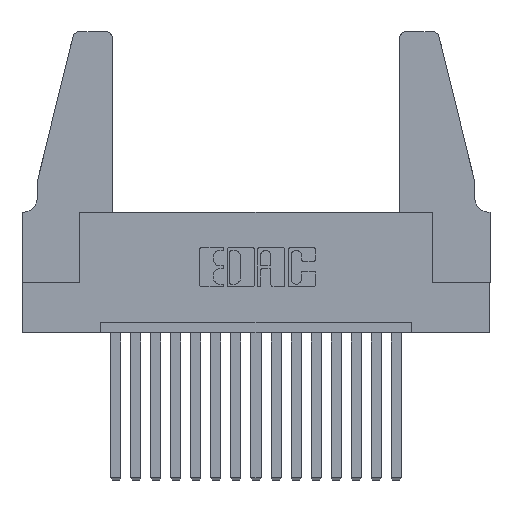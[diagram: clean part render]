
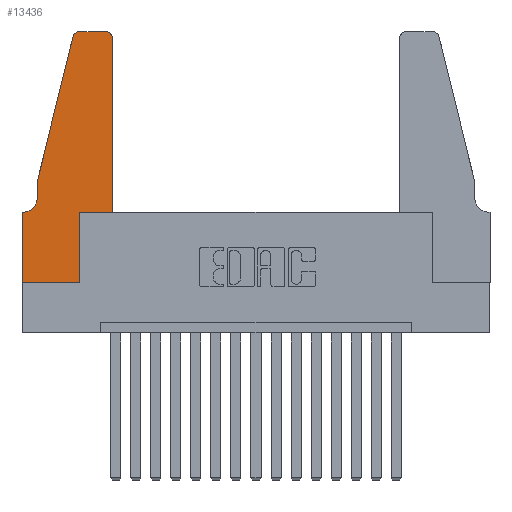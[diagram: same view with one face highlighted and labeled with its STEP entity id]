
A CAD part, top view. The second image highlights one B-rep face of the part: STEP entity #13436.
In plain terms, the highlighted planar face has unit normal (0, 0, 1).
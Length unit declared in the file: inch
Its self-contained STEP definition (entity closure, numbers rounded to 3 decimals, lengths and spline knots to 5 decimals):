
#142 = PLANE ( 'NONE',  #14912 ) ;
#301 = VERTEX_POINT ( 'NONE', #14000 ) ;
#553 = DIRECTION ( 'NONE',  ( 1., 0., 0. ) ) ;
#566 = ORIENTED_EDGE ( 'NONE', *, *, #6443, .T. ) ;
#1044 = DIRECTION ( 'NONE',  ( 1., 0., 0. ) ) ;
#1293 = VECTOR ( 'NONE', #553, 39.37008 ) ;
#1492 = VECTOR ( 'NONE', #10467, 39.37008 ) ;
#1547 = ORIENTED_EDGE ( 'NONE', *, *, #10667, .T. ) ;
#1606 = VECTOR ( 'NONE', #9524, 39.37008 ) ;
#1915 = LINE ( 'NONE', #5362, #1293 ) ;
#1996 = ORIENTED_EDGE ( 'NONE', *, *, #5969, .T. ) ;
#2199 = EDGE_CURVE ( 'NONE', #10345, #11494, #12308, .T. ) ;
#2483 = DIRECTION ( 'NONE',  ( 0., 0., -1. ) ) ;
#2499 = CARTESIAN_POINT ( 'NONE',  ( 0.2865, 0.35, 0.37 ) ) ;
#2780 = VERTEX_POINT ( 'NONE', #6485 ) ;
#2824 = CARTESIAN_POINT ( 'NONE',  ( 0.2865, 0.35, 0.37 ) ) ;
#2890 = CARTESIAN_POINT ( 'NONE',  ( 0.0755, 0.5, 0.37 ) ) ;
#3050 = EDGE_CURVE ( 'NONE', #11494, #301, #12895, .T. ) ;
#3321 = VECTOR ( 'NONE', #12921, 39.37008 ) ;
#3892 = VERTEX_POINT ( 'NONE', #12798 ) ;
#4064 = EDGE_CURVE ( 'NONE', #10422, #14339, #14464, .T. ) ;
#4308 = CARTESIAN_POINT ( 'NONE',  ( 0.2605, 1.25, 0.37 ) ) ;
#4333 = VECTOR ( 'NONE', #6754, 39.37008 ) ;
#4373 = CARTESIAN_POINT ( 'NONE',  ( 0., 0., 0.37 ) ) ;
#4433 = CARTESIAN_POINT ( 'NONE',  ( 0.0755, 0.35, 0.37 ) ) ;
#4600 = DIRECTION ( 'NONE',  ( 1., 0., 0. ) ) ;
#4766 = DIRECTION ( 'NONE',  ( 0., 0., 1. ) ) ;
#5066 = LINE ( 'NONE', #4308, #1606 ) ;
#5111 = EDGE_CURVE ( 'NONE', #3892, #8811, #5066, .T. ) ;
#5274 = EDGE_LOOP ( 'NONE', ( #10305, #7684, #6700, #5929, #566, #9186, #1996, #10435, #7729, #9344, #14558, #1547 ) ) ;
#5362 = CARTESIAN_POINT ( 'NONE',  ( 0., 0., 0.37 ) ) ;
#5525 = LINE ( 'NONE', #12229, #12070 ) ;
#5929 = ORIENTED_EDGE ( 'NONE', *, *, #3050, .T. ) ;
#5969 = EDGE_CURVE ( 'NONE', #14339, #2780, #11588, .T. ) ;
#6137 = CARTESIAN_POINT ( 'NONE',  ( 0.284, 1.25, 0.37 ) ) ;
#6207 = DIRECTION ( 'NONE',  ( 0., -1., 0. ) ) ;
#6263 = AXIS2_PLACEMENT_3D ( 'NONE', #7651, #6409, #1044 ) ;
#6409 = DIRECTION ( 'NONE',  ( 0., 0., 1. ) ) ;
#6429 = AXIS2_PLACEMENT_3D ( 'NONE', #16488, #4766, #4600 ) ;
#6443 = EDGE_CURVE ( 'NONE', #301, #10422, #11151, .T. ) ;
#6485 = CARTESIAN_POINT ( 'NONE',  ( 0., 0., 0.37 ) ) ;
#6700 = ORIENTED_EDGE ( 'NONE', *, *, #2199, .T. ) ;
#6754 = DIRECTION ( 'NONE',  ( 0., -1., 0. ) ) ;
#6848 = EDGE_CURVE ( 'NONE', #2780, #15087, #1915, .T. ) ;
#7066 = EDGE_CURVE ( 'NONE', #8811, #10345, #10366, .T. ) ;
#7296 = LINE ( 'NONE', #15345, #16460 ) ;
#7377 = CARTESIAN_POINT ( 'NONE',  ( 0.4505, 0.35, 0.37 ) ) ;
#7651 = CARTESIAN_POINT ( 'NONE',  ( 0.4205, 1.22, 0.37 ) ) ;
#7684 = ORIENTED_EDGE ( 'NONE', *, *, #7066, .T. ) ;
#7726 = DIRECTION ( 'NONE',  ( 0., 0., 1. ) ) ;
#7729 = ORIENTED_EDGE ( 'NONE', *, *, #11125, .T. ) ;
#8074 = VECTOR ( 'NONE', #6207, 39.37008 ) ;
#8448 = VERTEX_POINT ( 'NONE', #2824 ) ;
#8632 = CARTESIAN_POINT ( 'NONE',  ( 0.0055, 0.35, 0.37 ) ) ;
#8772 = DIRECTION ( 'NONE',  ( 1., 0., 0. ) ) ;
#8811 = VERTEX_POINT ( 'NONE', #6137 ) ;
#9153 = DIRECTION ( 'NONE',  ( 1., 0., 0. ) ) ;
#9186 = ORIENTED_EDGE ( 'NONE', *, *, #4064, .T. ) ;
#9344 = ORIENTED_EDGE ( 'NONE', *, *, #11722, .T. ) ;
#9485 = DIRECTION ( 'NONE',  ( -1., 0., 0. ) ) ;
#9524 = DIRECTION ( 'NONE',  ( -1., 0., 0. ) ) ;
#9608 = CIRCLE ( 'NONE', #6263, 0.03 ) ;
#9613 = CARTESIAN_POINT ( 'NONE',  ( 0., 0.35, 0.37 ) ) ;
#10305 = ORIENTED_EDGE ( 'NONE', *, *, #5111, .T. ) ;
#10307 = VERTEX_POINT ( 'NONE', #7377 ) ;
#10345 = VERTEX_POINT ( 'NONE', #15296 ) ;
#10366 = CIRCLE ( 'NONE', #6429, 0.03 ) ;
#10391 = CARTESIAN_POINT ( 'NONE',  ( 0.0055, 0.42, 0.37 ) ) ;
#10422 = VERTEX_POINT ( 'NONE', #8632 ) ;
#10435 = ORIENTED_EDGE ( 'NONE', *, *, #6848, .T. ) ;
#10467 = DIRECTION ( 'NONE',  ( -0.239, -0.971, 0. ) ) ;
#10667 = EDGE_CURVE ( 'NONE', #12826, #3892, #9608, .T. ) ;
#11125 = EDGE_CURVE ( 'NONE', #15087, #8448, #11662, .T. ) ;
#11151 = CIRCLE ( 'NONE', #16036, 0.07 ) ;
#11494 = VERTEX_POINT ( 'NONE', #2890 ) ;
#11588 = LINE ( 'NONE', #4373, #8074 ) ;
#11662 = LINE ( 'NONE', #2499, #3321 ) ;
#11699 = CARTESIAN_POINT ( 'NONE',  ( 0., 0.35, 0.37 ) ) ;
#11722 = EDGE_CURVE ( 'NONE', #8448, #10307, #5525, .T. ) ;
#12070 = VECTOR ( 'NONE', #8772, 39.37008 ) ;
#12220 = CARTESIAN_POINT ( 'NONE',  ( 0.4505, 1.22, 0.37 ) ) ;
#12229 = CARTESIAN_POINT ( 'NONE',  ( 0.4505, 0.35, 0.37 ) ) ;
#12308 = LINE ( 'NONE', #15869, #1492 ) ;
#12798 = CARTESIAN_POINT ( 'NONE',  ( 0.4205, 1.25, 0.37 ) ) ;
#12826 = VERTEX_POINT ( 'NONE', #12220 ) ;
#12895 = LINE ( 'NONE', #15818, #4333 ) ;
#12921 = DIRECTION ( 'NONE',  ( 0., 1., 0. ) ) ;
#13436 = ADVANCED_FACE ( 'NONE', ( #13996 ), #142, .T. ) ;
#13996 = FACE_OUTER_BOUND ( 'NONE', #5274, .T. ) ;
#14000 = CARTESIAN_POINT ( 'NONE',  ( 0.0755, 0.42, 0.37 ) ) ;
#14024 = DIRECTION ( 'NONE',  ( -1., 0., 0. ) ) ;
#14339 = VERTEX_POINT ( 'NONE', #9613 ) ;
#14464 = LINE ( 'NONE', #4433, #15059 ) ;
#14558 = ORIENTED_EDGE ( 'NONE', *, *, #16816, .T. ) ;
#14912 = AXIS2_PLACEMENT_3D ( 'NONE', #11699, #7726, #9153 ) ;
#14988 = CARTESIAN_POINT ( 'NONE',  ( 0.2865, 0., 0.37 ) ) ;
#15059 = VECTOR ( 'NONE', #9485, 39.37008 ) ;
#15087 = VERTEX_POINT ( 'NONE', #14988 ) ;
#15296 = CARTESIAN_POINT ( 'NONE',  ( 0.25487, 1.22718, 0.37 ) ) ;
#15345 = CARTESIAN_POINT ( 'NONE',  ( 0.4505, 0.35, 0.37 ) ) ;
#15588 = DIRECTION ( 'NONE',  ( 0., 1., 0. ) ) ;
#15818 = CARTESIAN_POINT ( 'NONE',  ( 0.0755, 0.5, 0.37 ) ) ;
#15869 = CARTESIAN_POINT ( 'NONE',  ( 0.0755, 0.5, 0.37 ) ) ;
#16036 = AXIS2_PLACEMENT_3D ( 'NONE', #10391, #2483, #14024 ) ;
#16460 = VECTOR ( 'NONE', #15588, 39.37008 ) ;
#16488 = CARTESIAN_POINT ( 'NONE',  ( 0.284, 1.22, 0.37 ) ) ;
#16816 = EDGE_CURVE ( 'NONE', #10307, #12826, #7296, .T. ) ;
